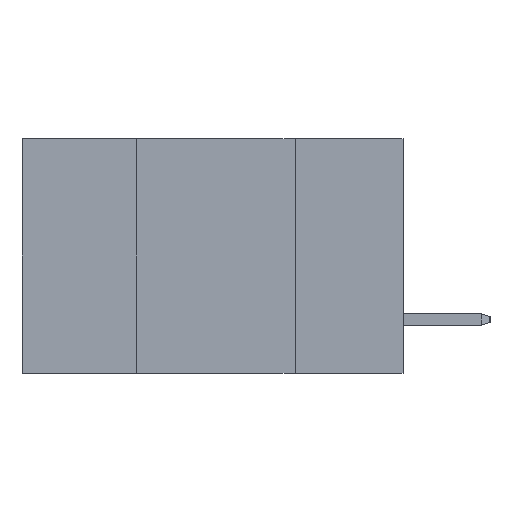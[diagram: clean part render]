
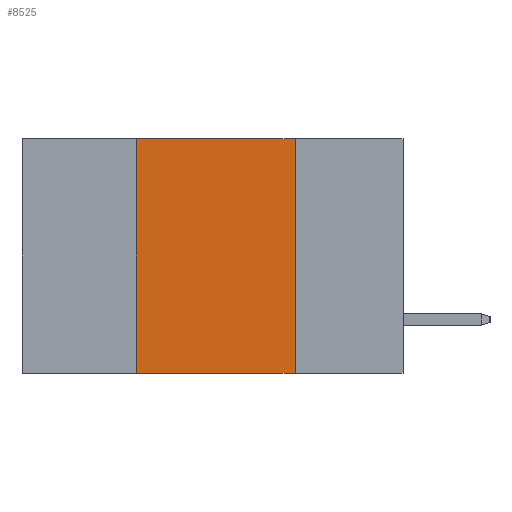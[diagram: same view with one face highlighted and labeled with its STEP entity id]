
A CAD part, left-side view. The second image highlights one B-rep face of the part: STEP entity #8525.
In plain terms, the highlighted planar face has unit normal (-1, 0, 0).
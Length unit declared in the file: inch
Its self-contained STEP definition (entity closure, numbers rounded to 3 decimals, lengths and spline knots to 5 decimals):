
#116 = VECTOR ( 'NONE', #5972, 39.37008 ) ;
#167 = VECTOR ( 'NONE', #7938, 39.37008 ) ;
#246 = LINE ( 'NONE', #1121, #167 ) ;
#283 = EDGE_CURVE ( 'NONE', #11810, #10348, #4875, .T. ) ;
#1121 = CARTESIAN_POINT ( 'NONE',  ( 0., 0.6, 0. ) ) ;
#1612 = VECTOR ( 'NONE', #11511, 39.37008 ) ;
#1684 = CARTESIAN_POINT ( 'NONE',  ( 0., 0.17, 0. ) ) ;
#2037 = EDGE_LOOP ( 'NONE', ( #2507, #2040, #7273, #8106 ) ) ;
#2040 = ORIENTED_EDGE ( 'NONE', *, *, #7190, .F. ) ;
#2507 = ORIENTED_EDGE ( 'NONE', *, *, #9642, .F. ) ;
#3254 = VECTOR ( 'NONE', #7682, 39.37008 ) ;
#3609 = VERTEX_POINT ( 'NONE', #12155 ) ;
#4875 = LINE ( 'NONE', #6739, #116 ) ;
#5922 = AXIS2_PLACEMENT_3D ( 'NONE', #9862, #11919, #6137 ) ;
#5972 = DIRECTION ( 'NONE',  ( 0., 0., 1. ) ) ;
#6137 = DIRECTION ( 'NONE',  ( 0., 0., -1. ) ) ;
#6203 = FACE_OUTER_BOUND ( 'NONE', #2037, .T. ) ;
#6739 = CARTESIAN_POINT ( 'NONE',  ( 0., 0.42, 0. ) ) ;
#7190 = EDGE_CURVE ( 'NONE', #10348, #7580, #246, .T. ) ;
#7193 = CARTESIAN_POINT ( 'NONE',  ( 0., 0.42, -0.37 ) ) ;
#7273 = ORIENTED_EDGE ( 'NONE', *, *, #283, .F. ) ;
#7580 = VERTEX_POINT ( 'NONE', #1684 ) ;
#7682 = DIRECTION ( 'NONE',  ( 0., 0., -1. ) ) ;
#7798 = LINE ( 'NONE', #10483, #1612 ) ;
#7849 = CARTESIAN_POINT ( 'NONE',  ( 0., 0.42, 0. ) ) ;
#7938 = DIRECTION ( 'NONE',  ( 0., -1., 0. ) ) ;
#8106 = ORIENTED_EDGE ( 'NONE', *, *, #8716, .T. ) ;
#8525 = ADVANCED_FACE ( 'NONE', ( #6203 ), #11979, .F. ) ;
#8716 = EDGE_CURVE ( 'NONE', #11810, #3609, #7798, .T. ) ;
#9642 = EDGE_CURVE ( 'NONE', #7580, #3609, #10746, .T. ) ;
#9862 = CARTESIAN_POINT ( 'NONE',  ( 0., 0.6, 0. ) ) ;
#10348 = VERTEX_POINT ( 'NONE', #7849 ) ;
#10483 = CARTESIAN_POINT ( 'NONE',  ( 0., 0.6, -0.37 ) ) ;
#10746 = LINE ( 'NONE', #11654, #3254 ) ;
#11511 = DIRECTION ( 'NONE',  ( 0., -1., 0. ) ) ;
#11654 = CARTESIAN_POINT ( 'NONE',  ( 0., 0.17, 0. ) ) ;
#11810 = VERTEX_POINT ( 'NONE', #7193 ) ;
#11919 = DIRECTION ( 'NONE',  ( 1., 0., 0. ) ) ;
#11979 = PLANE ( 'NONE',  #5922 ) ;
#12155 = CARTESIAN_POINT ( 'NONE',  ( 0., 0.17, -0.37 ) ) ;
